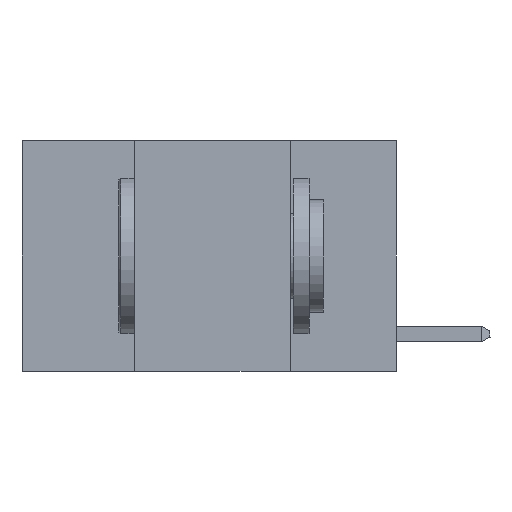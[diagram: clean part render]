
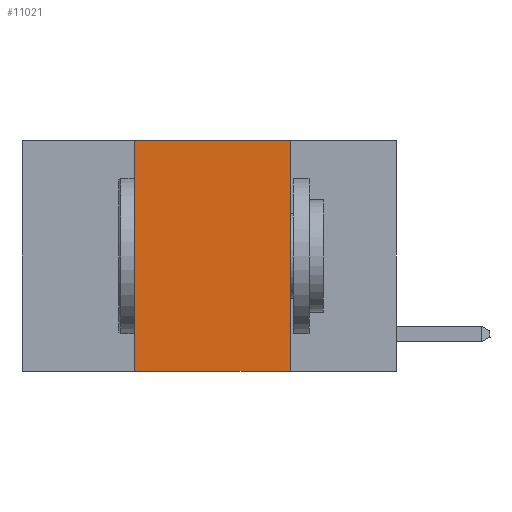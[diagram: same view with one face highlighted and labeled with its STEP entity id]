
A CAD part, left-side view. The second image highlights one B-rep face of the part: STEP entity #11021.
In plain terms, the highlighted planar face has unit normal (-1, 0, 0).
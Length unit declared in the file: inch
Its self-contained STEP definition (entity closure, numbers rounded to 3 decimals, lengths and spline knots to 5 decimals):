
#575 = VERTEX_POINT ( 'NONE', #17092 ) ;
#1381 = EDGE_CURVE ( 'NONE', #6549, #19307, #9596, .T. ) ;
#1839 = VERTEX_POINT ( 'NONE', #16885 ) ;
#3566 = DIRECTION ( 'NONE',  ( 1., 0., 0. ) ) ;
#3745 = EDGE_CURVE ( 'NONE', #6549, #575, #20013, .T. ) ;
#3766 = CARTESIAN_POINT ( 'NONE',  ( 0., 0.17, -0.37 ) ) ;
#4200 = EDGE_LOOP ( 'NONE', ( #12566, #22333, #10669, #20422 ) ) ;
#4234 = DIRECTION ( 'NONE',  ( 0., 0., -1. ) ) ;
#6258 = AXIS2_PLACEMENT_3D ( 'NONE', #14056, #3566, #15812 ) ;
#6549 = VERTEX_POINT ( 'NONE', #13049 ) ;
#7022 = PLANE ( 'NONE',  #6258 ) ;
#7921 = VECTOR ( 'NONE', #4234, 39.37008 ) ;
#8008 = LINE ( 'NONE', #22338, #21831 ) ;
#8394 = FACE_OUTER_BOUND ( 'NONE', #4200, .T. ) ;
#9185 = CARTESIAN_POINT ( 'NONE',  ( 0., 0.6, -0.37 ) ) ;
#9596 = LINE ( 'NONE', #9185, #21794 ) ;
#10669 = ORIENTED_EDGE ( 'NONE', *, *, #3745, .F. ) ;
#11021 = ADVANCED_FACE ( 'NONE', ( #8394 ), #7022, .F. ) ;
#11194 = CARTESIAN_POINT ( 'NONE',  ( 0., 0.17, 0. ) ) ;
#11958 = DIRECTION ( 'NONE',  ( 0., -1., 0. ) ) ;
#12566 = ORIENTED_EDGE ( 'NONE', *, *, #20095, .F. ) ;
#13049 = CARTESIAN_POINT ( 'NONE',  ( 0., 0.42, -0.37 ) ) ;
#14056 = CARTESIAN_POINT ( 'NONE',  ( 0., 0.6, 0. ) ) ;
#14152 = EDGE_CURVE ( 'NONE', #575, #1839, #8008, .T. ) ;
#15443 = VECTOR ( 'NONE', #16582, 39.37008 ) ;
#15812 = DIRECTION ( 'NONE',  ( 0., 0., -1. ) ) ;
#16582 = DIRECTION ( 'NONE',  ( 0., 0., 1. ) ) ;
#16885 = CARTESIAN_POINT ( 'NONE',  ( 0., 0.17, 0. ) ) ;
#17092 = CARTESIAN_POINT ( 'NONE',  ( 0., 0.42, 0. ) ) ;
#17729 = LINE ( 'NONE', #11194, #7921 ) ;
#18531 = DIRECTION ( 'NONE',  ( 0., -1., 0. ) ) ;
#19307 = VERTEX_POINT ( 'NONE', #3766 ) ;
#19961 = CARTESIAN_POINT ( 'NONE',  ( 0., 0.42, 0. ) ) ;
#20013 = LINE ( 'NONE', #19961, #15443 ) ;
#20095 = EDGE_CURVE ( 'NONE', #1839, #19307, #17729, .T. ) ;
#20422 = ORIENTED_EDGE ( 'NONE', *, *, #1381, .T. ) ;
#21794 = VECTOR ( 'NONE', #18531, 39.37008 ) ;
#21831 = VECTOR ( 'NONE', #11958, 39.37008 ) ;
#22333 = ORIENTED_EDGE ( 'NONE', *, *, #14152, .F. ) ;
#22338 = CARTESIAN_POINT ( 'NONE',  ( 0., 0.6, 0. ) ) ;
